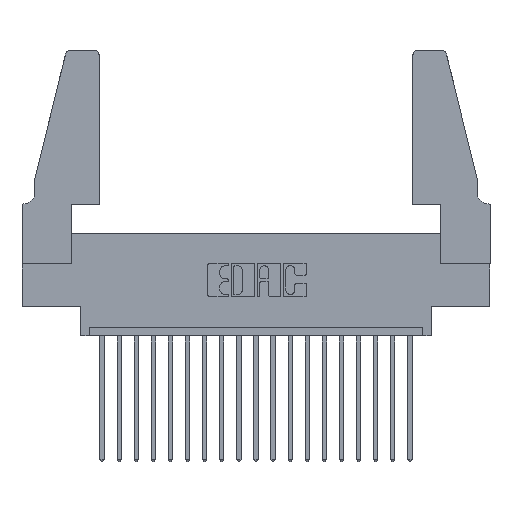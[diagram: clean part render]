
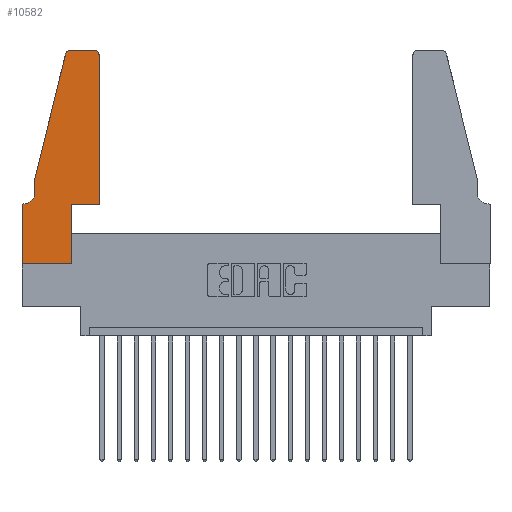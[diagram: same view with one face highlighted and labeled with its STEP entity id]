
A CAD part, top view. The second image highlights one B-rep face of the part: STEP entity #10582.
In plain terms, the highlighted planar face has unit normal (0, 0, 1).
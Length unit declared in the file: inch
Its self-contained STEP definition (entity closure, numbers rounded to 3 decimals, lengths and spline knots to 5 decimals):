
#718 = PLANE ( 'NONE',  #7016 ) ;
#836 = EDGE_CURVE ( 'NONE', #2809, #6692, #5040, .T. ) ;
#866 = DIRECTION ( 'NONE',  ( 0., -1., 0. ) ) ;
#1205 = VECTOR ( 'NONE', #8222, 39.37008 ) ;
#1371 = VECTOR ( 'NONE', #7659, 39.37008 ) ;
#1477 = VECTOR ( 'NONE', #3928, 39.37008 ) ;
#1534 = LINE ( 'NONE', #18651, #6501 ) ;
#1561 = EDGE_CURVE ( 'NONE', #11456, #11125, #6195, .T. ) ;
#1580 = CARTESIAN_POINT ( 'NONE',  ( 0.4505, 0.35, 0.37 ) ) ;
#2531 = CARTESIAN_POINT ( 'NONE',  ( 0.4505, 0.35, 0.37 ) ) ;
#2590 = CARTESIAN_POINT ( 'NONE',  ( 0.0055, 0.42, 0.37 ) ) ;
#2729 = CARTESIAN_POINT ( 'NONE',  ( 0., 0., 0.37 ) ) ;
#2809 = VERTEX_POINT ( 'NONE', #7719 ) ;
#2818 = AXIS2_PLACEMENT_3D ( 'NONE', #18208, #7842, #14051 ) ;
#3266 = CIRCLE ( 'NONE', #11218, 0.07 ) ;
#3305 = VERTEX_POINT ( 'NONE', #2729 ) ;
#3412 = EDGE_CURVE ( 'NONE', #8897, #18920, #5395, .T. ) ;
#3758 = CARTESIAN_POINT ( 'NONE',  ( 0., 0.35, 0.37 ) ) ;
#3928 = DIRECTION ( 'NONE',  ( 0., 1., 0. ) ) ;
#4068 = EDGE_CURVE ( 'NONE', #18920, #13769, #6415, .T. ) ;
#4104 = DIRECTION ( 'NONE',  ( 0., 0., -1. ) ) ;
#4154 = LINE ( 'NONE', #17624, #15836 ) ;
#4389 = EDGE_CURVE ( 'NONE', #13769, #11456, #19318, .T. ) ;
#4450 = ORIENTED_EDGE ( 'NONE', *, *, #15918, .T. ) ;
#4571 = ORIENTED_EDGE ( 'NONE', *, *, #1561, .T. ) ;
#4971 = LINE ( 'NONE', #13843, #17838 ) ;
#5040 = CIRCLE ( 'NONE', #16722, 0.03 ) ;
#5140 = EDGE_CURVE ( 'NONE', #3305, #8897, #18092, .T. ) ;
#5360 = VECTOR ( 'NONE', #18262, 39.37008 ) ;
#5395 = LINE ( 'NONE', #5861, #1371 ) ;
#5500 = ORIENTED_EDGE ( 'NONE', *, *, #14306, .T. ) ;
#5508 = CARTESIAN_POINT ( 'NONE',  ( 0.0755, 0.35, 0.37 ) ) ;
#5861 = CARTESIAN_POINT ( 'NONE',  ( 0.2865, 0.35, 0.37 ) ) ;
#5952 = ORIENTED_EDGE ( 'NONE', *, *, #3412, .T. ) ;
#6195 = CIRCLE ( 'NONE', #2818, 0.03 ) ;
#6408 = CARTESIAN_POINT ( 'NONE',  ( 0.2605, 1.25, 0.37 ) ) ;
#6415 = LINE ( 'NONE', #1580, #18099 ) ;
#6501 = VECTOR ( 'NONE', #11446, 39.37008 ) ;
#6529 = VECTOR ( 'NONE', #10263, 39.37008 ) ;
#6692 = VERTEX_POINT ( 'NONE', #8638 ) ;
#7013 = CARTESIAN_POINT ( 'NONE',  ( 0., 0.35, 0.37 ) ) ;
#7016 = AXIS2_PLACEMENT_3D ( 'NONE', #3758, #15947, #9900 ) ;
#7276 = VERTEX_POINT ( 'NONE', #9030 ) ;
#7630 = ORIENTED_EDGE ( 'NONE', *, *, #10446, .T. ) ;
#7659 = DIRECTION ( 'NONE',  ( 0., 1., 0. ) ) ;
#7719 = CARTESIAN_POINT ( 'NONE',  ( 0.284, 1.25, 0.37 ) ) ;
#7842 = DIRECTION ( 'NONE',  ( 0., 0., 1. ) ) ;
#8222 = DIRECTION ( 'NONE',  ( 1., 0., 0. ) ) ;
#8638 = CARTESIAN_POINT ( 'NONE',  ( 0.25487, 1.22718, 0.37 ) ) ;
#8897 = VERTEX_POINT ( 'NONE', #19593 ) ;
#8925 = ORIENTED_EDGE ( 'NONE', *, *, #5140, .T. ) ;
#9030 = CARTESIAN_POINT ( 'NONE',  ( 0.0755, 0.42, 0.37 ) ) ;
#9238 = ORIENTED_EDGE ( 'NONE', *, *, #4068, .T. ) ;
#9367 = CARTESIAN_POINT ( 'NONE',  ( 0.4505, 1.22, 0.37 ) ) ;
#9404 = ORIENTED_EDGE ( 'NONE', *, *, #16819, .T. ) ;
#9900 = DIRECTION ( 'NONE',  ( 1., 0., 0. ) ) ;
#10263 = DIRECTION ( 'NONE',  ( -1., 0., 0. ) ) ;
#10446 = EDGE_CURVE ( 'NONE', #6692, #17704, #1534, .T. ) ;
#10481 = CARTESIAN_POINT ( 'NONE',  ( 0.2865, 0.35, 0.37 ) ) ;
#10582 = ADVANCED_FACE ( 'NONE', ( #12026 ), #718, .T. ) ;
#11125 = VERTEX_POINT ( 'NONE', #19705 ) ;
#11218 = AXIS2_PLACEMENT_3D ( 'NONE', #2590, #4104, #14786 ) ;
#11446 = DIRECTION ( 'NONE',  ( -0.239, -0.971, 0. ) ) ;
#11456 = VERTEX_POINT ( 'NONE', #9367 ) ;
#11735 = ORIENTED_EDGE ( 'NONE', *, *, #836, .T. ) ;
#12026 = FACE_OUTER_BOUND ( 'NONE', #18235, .T. ) ;
#12523 = LINE ( 'NONE', #5508, #6529 ) ;
#12685 = EDGE_CURVE ( 'NONE', #16582, #3305, #4971, .T. ) ;
#13505 = CARTESIAN_POINT ( 'NONE',  ( 0.0755, 0.5, 0.37 ) ) ;
#13537 = ORIENTED_EDGE ( 'NONE', *, *, #4389, .T. ) ;
#13639 = DIRECTION ( 'NONE',  ( 1., 0., 0. ) ) ;
#13769 = VERTEX_POINT ( 'NONE', #14549 ) ;
#13843 = CARTESIAN_POINT ( 'NONE',  ( 0., 0., 0.37 ) ) ;
#13855 = CARTESIAN_POINT ( 'NONE',  ( 0.0055, 0.35, 0.37 ) ) ;
#13910 = VERTEX_POINT ( 'NONE', #13855 ) ;
#14051 = DIRECTION ( 'NONE',  ( 1., 0., 0. ) ) ;
#14306 = EDGE_CURVE ( 'NONE', #7276, #13910, #3266, .T. ) ;
#14439 = ORIENTED_EDGE ( 'NONE', *, *, #12685, .T. ) ;
#14549 = CARTESIAN_POINT ( 'NONE',  ( 0.4505, 0.35, 0.37 ) ) ;
#14583 = DIRECTION ( 'NONE',  ( 0., 0., 1. ) ) ;
#14786 = DIRECTION ( 'NONE',  ( -1., 0., 0. ) ) ;
#14844 = DIRECTION ( 'NONE',  ( 1., 0., 0. ) ) ;
#15305 = DIRECTION ( 'NONE',  ( 0., -1., 0. ) ) ;
#15836 = VECTOR ( 'NONE', #866, 39.37008 ) ;
#15918 = EDGE_CURVE ( 'NONE', #17704, #7276, #4154, .T. ) ;
#15947 = DIRECTION ( 'NONE',  ( 0., 0., 1. ) ) ;
#16051 = EDGE_CURVE ( 'NONE', #13910, #16582, #12523, .T. ) ;
#16582 = VERTEX_POINT ( 'NONE', #7013 ) ;
#16722 = AXIS2_PLACEMENT_3D ( 'NONE', #17795, #14583, #14844 ) ;
#16819 = EDGE_CURVE ( 'NONE', #11125, #2809, #18940, .T. ) ;
#16892 = ORIENTED_EDGE ( 'NONE', *, *, #16051, .T. ) ;
#17624 = CARTESIAN_POINT ( 'NONE',  ( 0.0755, 0.5, 0.37 ) ) ;
#17704 = VERTEX_POINT ( 'NONE', #13505 ) ;
#17795 = CARTESIAN_POINT ( 'NONE',  ( 0.284, 1.22, 0.37 ) ) ;
#17838 = VECTOR ( 'NONE', #15305, 39.37008 ) ;
#18092 = LINE ( 'NONE', #18589, #1205 ) ;
#18099 = VECTOR ( 'NONE', #13639, 39.37008 ) ;
#18208 = CARTESIAN_POINT ( 'NONE',  ( 0.4205, 1.22, 0.37 ) ) ;
#18235 = EDGE_LOOP ( 'NONE', ( #9404, #11735, #7630, #4450, #5500, #16892, #14439, #8925, #5952, #9238, #13537, #4571 ) ) ;
#18262 = DIRECTION ( 'NONE',  ( -1., 0., 0. ) ) ;
#18589 = CARTESIAN_POINT ( 'NONE',  ( 0., 0., 0.37 ) ) ;
#18651 = CARTESIAN_POINT ( 'NONE',  ( 0.0755, 0.5, 0.37 ) ) ;
#18920 = VERTEX_POINT ( 'NONE', #10481 ) ;
#18940 = LINE ( 'NONE', #6408, #5360 ) ;
#19318 = LINE ( 'NONE', #2531, #1477 ) ;
#19593 = CARTESIAN_POINT ( 'NONE',  ( 0.2865, 0., 0.37 ) ) ;
#19705 = CARTESIAN_POINT ( 'NONE',  ( 0.4205, 1.25, 0.37 ) ) ;
